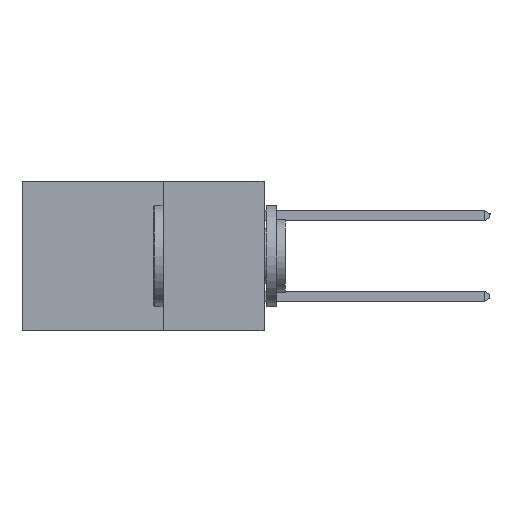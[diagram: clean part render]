
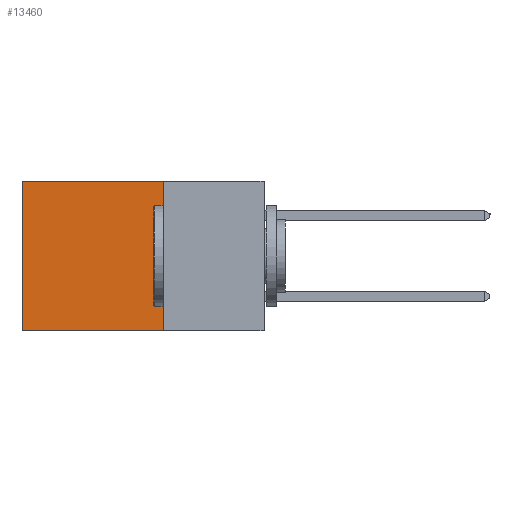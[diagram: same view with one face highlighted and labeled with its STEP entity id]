
A CAD part, left-side view. The second image highlights one B-rep face of the part: STEP entity #13460.
In plain terms, the highlighted planar face has unit normal (-1, 0, 0).
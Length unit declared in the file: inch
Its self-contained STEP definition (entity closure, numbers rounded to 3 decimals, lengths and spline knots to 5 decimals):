
#1204 = ORIENTED_EDGE ( 'NONE', *, *, #5545, .T. ) ;
#1236 = VERTEX_POINT ( 'NONE', #2612 ) ;
#1879 = VERTEX_POINT ( 'NONE', #2947 ) ;
#2612 = CARTESIAN_POINT ( 'NONE',  ( 0.2615, 0.6, -0.37 ) ) ;
#2723 = CARTESIAN_POINT ( 'NONE',  ( 0.2615, 0.25, -0.37 ) ) ;
#2947 = CARTESIAN_POINT ( 'NONE',  ( 0.2615, 0.6, 0. ) ) ;
#3255 = CARTESIAN_POINT ( 'NONE',  ( 0.2615, 0.6, -0.37 ) ) ;
#3615 = VECTOR ( 'NONE', #13908, 39.37008 ) ;
#3740 = CARTESIAN_POINT ( 'NONE',  ( 0.2615, 0.25, 0. ) ) ;
#3898 = ORIENTED_EDGE ( 'NONE', *, *, #10323, .F. ) ;
#5229 = DIRECTION ( 'NONE',  ( 0., 0., -1. ) ) ;
#5297 = VECTOR ( 'NONE', #5229, 39.37008 ) ;
#5545 = EDGE_CURVE ( 'NONE', #9702, #1879, #8172, .T. ) ;
#6113 = DIRECTION ( 'NONE',  ( 0., 0., -1. ) ) ;
#6195 = DIRECTION ( 'NONE',  ( 1., 0., 0. ) ) ;
#6349 = LINE ( 'NONE', #7715, #9065 ) ;
#6689 = LINE ( 'NONE', #11981, #5297 ) ;
#7084 = ORIENTED_EDGE ( 'NONE', *, *, #7834, .F. ) ;
#7408 = FACE_OUTER_BOUND ( 'NONE', #11028, .T. ) ;
#7518 = VECTOR ( 'NONE', #9737, 39.37008 ) ;
#7552 = LINE ( 'NONE', #3255, #7518 ) ;
#7715 = CARTESIAN_POINT ( 'NONE',  ( 0.2615, 0.25, -0.37 ) ) ;
#7834 = EDGE_CURVE ( 'NONE', #9702, #9686, #6689, .T. ) ;
#8172 = LINE ( 'NONE', #3740, #3615 ) ;
#9065 = VECTOR ( 'NONE', #10777, 39.37008 ) ;
#9136 = AXIS2_PLACEMENT_3D ( 'NONE', #14101, #6195, #6113 ) ;
#9686 = VERTEX_POINT ( 'NONE', #2723 ) ;
#9702 = VERTEX_POINT ( 'NONE', #12098 ) ;
#9737 = DIRECTION ( 'NONE',  ( 0., 0., -1. ) ) ;
#10323 = EDGE_CURVE ( 'NONE', #9686, #1236, #6349, .T. ) ;
#10777 = DIRECTION ( 'NONE',  ( 0., 1., 0. ) ) ;
#11028 = EDGE_LOOP ( 'NONE', ( #12764, #3898, #7084, #1204 ) ) ;
#11981 = CARTESIAN_POINT ( 'NONE',  ( 0.2615, 0.25, -0.37 ) ) ;
#12098 = CARTESIAN_POINT ( 'NONE',  ( 0.2615, 0.25, 0. ) ) ;
#12307 = EDGE_CURVE ( 'NONE', #1879, #1236, #7552, .T. ) ;
#12764 = ORIENTED_EDGE ( 'NONE', *, *, #12307, .T. ) ;
#13460 = ADVANCED_FACE ( 'NONE', ( #7408 ), #14022, .F. ) ;
#13908 = DIRECTION ( 'NONE',  ( 0., 1., 0. ) ) ;
#14022 = PLANE ( 'NONE',  #9136 ) ;
#14101 = CARTESIAN_POINT ( 'NONE',  ( 0.2615, 0.25, -0.37 ) ) ;
